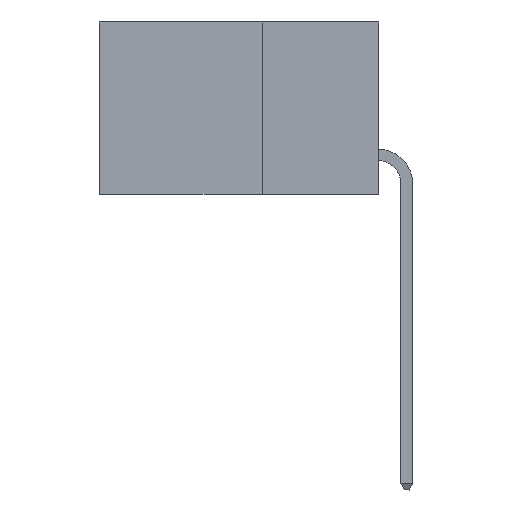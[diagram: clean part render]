
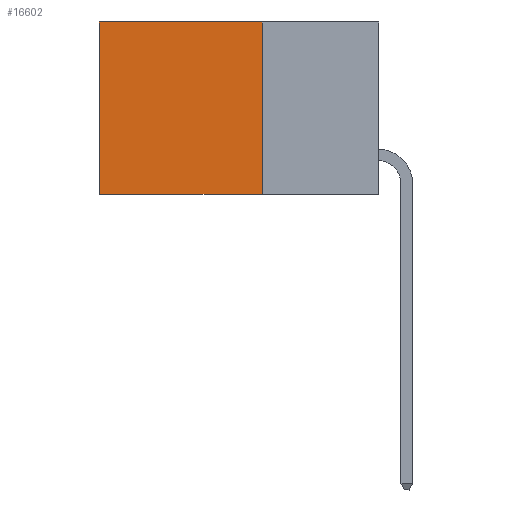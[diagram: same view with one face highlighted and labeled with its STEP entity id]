
A CAD part, left-side view. The second image highlights one B-rep face of the part: STEP entity #16602.
In plain terms, the highlighted planar face has unit normal (-1, 0, 0).
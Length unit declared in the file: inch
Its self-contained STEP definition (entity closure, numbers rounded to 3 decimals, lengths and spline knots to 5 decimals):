
#312 = CARTESIAN_POINT ( 'NONE',  ( 0.2615, 0.25, -0.37 ) ) ;
#625 = DIRECTION ( 'NONE',  ( 0., 1., 0. ) ) ;
#3212 = CARTESIAN_POINT ( 'NONE',  ( 0.2615, 0.6, -0.37 ) ) ;
#4357 = VERTEX_POINT ( 'NONE', #3212 ) ;
#4698 = PLANE ( 'NONE',  #15241 ) ;
#4909 = LINE ( 'NONE', #18159, #17955 ) ;
#5097 = ORIENTED_EDGE ( 'NONE', *, *, #7246, .T. ) ;
#5869 = DIRECTION ( 'NONE',  ( 0., 0., -1. ) ) ;
#5968 = LINE ( 'NONE', #11833, #12064 ) ;
#6241 = DIRECTION ( 'NONE',  ( 1., 0., 0. ) ) ;
#7090 = LINE ( 'NONE', #13057, #16158 ) ;
#7246 = EDGE_CURVE ( 'NONE', #18301, #10346, #7090, .T. ) ;
#9074 = CARTESIAN_POINT ( 'NONE',  ( 0.2615, 0.6, -0.37 ) ) ;
#10346 = VERTEX_POINT ( 'NONE', #15611 ) ;
#11214 = EDGE_CURVE ( 'NONE', #18301, #12040, #5968, .T. ) ;
#11825 = CARTESIAN_POINT ( 'NONE',  ( 0.2615, 0.25, -0.37 ) ) ;
#11833 = CARTESIAN_POINT ( 'NONE',  ( 0.2615, 0.25, -0.37 ) ) ;
#12039 = ORIENTED_EDGE ( 'NONE', *, *, #14645, .F. ) ;
#12040 = VERTEX_POINT ( 'NONE', #312 ) ;
#12064 = VECTOR ( 'NONE', #12215, 39.37008 ) ;
#12215 = DIRECTION ( 'NONE',  ( 0., 0., -1. ) ) ;
#12855 = DIRECTION ( 'NONE',  ( 0., 1., 0. ) ) ;
#13057 = CARTESIAN_POINT ( 'NONE',  ( 0.2615, 0.25, 0. ) ) ;
#13393 = LINE ( 'NONE', #9074, #16434 ) ;
#14315 = EDGE_LOOP ( 'NONE', ( #15043, #12039, #16624, #5097 ) ) ;
#14645 = EDGE_CURVE ( 'NONE', #12040, #4357, #4909, .T. ) ;
#14935 = DIRECTION ( 'NONE',  ( 0., 0., -1. ) ) ;
#15043 = ORIENTED_EDGE ( 'NONE', *, *, #15460, .T. ) ;
#15241 = AXIS2_PLACEMENT_3D ( 'NONE', #11825, #6241, #5869 ) ;
#15460 = EDGE_CURVE ( 'NONE', #10346, #4357, #13393, .T. ) ;
#15611 = CARTESIAN_POINT ( 'NONE',  ( 0.2615, 0.6, 0. ) ) ;
#16158 = VECTOR ( 'NONE', #12855, 39.37008 ) ;
#16247 = FACE_OUTER_BOUND ( 'NONE', #14315, .T. ) ;
#16434 = VECTOR ( 'NONE', #14935, 39.37008 ) ;
#16602 = ADVANCED_FACE ( 'NONE', ( #16247 ), #4698, .F. ) ;
#16624 = ORIENTED_EDGE ( 'NONE', *, *, #11214, .F. ) ;
#17572 = CARTESIAN_POINT ( 'NONE',  ( 0.2615, 0.25, 0. ) ) ;
#17955 = VECTOR ( 'NONE', #625, 39.37008 ) ;
#18159 = CARTESIAN_POINT ( 'NONE',  ( 0.2615, 0.25, -0.37 ) ) ;
#18301 = VERTEX_POINT ( 'NONE', #17572 ) ;
